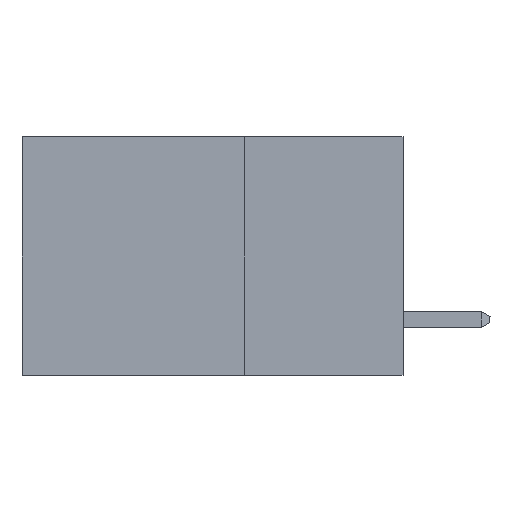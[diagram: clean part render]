
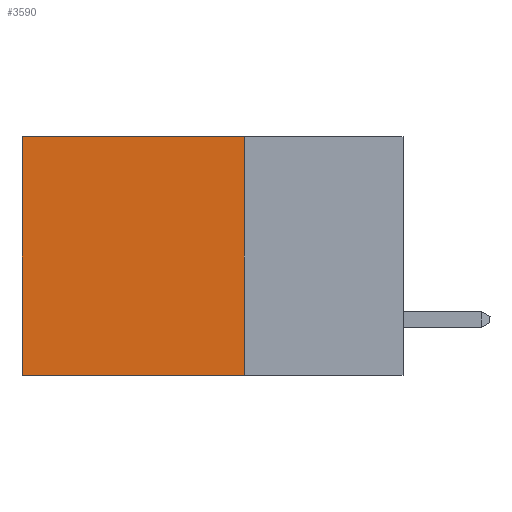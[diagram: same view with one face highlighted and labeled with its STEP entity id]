
A CAD part, left-side view. The second image highlights one B-rep face of the part: STEP entity #3590.
In plain terms, the highlighted planar face has unit normal (-1, 0, 0).
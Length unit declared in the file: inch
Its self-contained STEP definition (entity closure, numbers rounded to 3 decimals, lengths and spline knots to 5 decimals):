
#98 = VECTOR ( 'NONE', #6713, 39.37008 ) ;
#166 = VERTEX_POINT ( 'NONE', #9042 ) ;
#583 = LINE ( 'NONE', #1980, #8184 ) ;
#744 = VECTOR ( 'NONE', #755, 39.37008 ) ;
#755 = DIRECTION ( 'NONE',  ( 0., 0., -1. ) ) ;
#811 = EDGE_LOOP ( 'NONE', ( #7023, #7026, #1239, #4634 ) ) ;
#1239 = ORIENTED_EDGE ( 'NONE', *, *, #2025, .F. ) ;
#1556 = CARTESIAN_POINT ( 'NONE',  ( 0.2875, 0.25, -0.375 ) ) ;
#1712 = VERTEX_POINT ( 'NONE', #8568 ) ;
#1980 = CARTESIAN_POINT ( 'NONE',  ( 0.2875, 0.25, -0.375 ) ) ;
#2025 = EDGE_CURVE ( 'NONE', #3100, #166, #4269, .T. ) ;
#2081 = DIRECTION ( 'NONE',  ( 1., 0., 0. ) ) ;
#2112 = CARTESIAN_POINT ( 'NONE',  ( 0.2875, 0.6, -0.375 ) ) ;
#2979 = CARTESIAN_POINT ( 'NONE',  ( 0.2875, 0.25, 0. ) ) ;
#3008 = EDGE_CURVE ( 'NONE', #3100, #6334, #3666, .T. ) ;
#3100 = VERTEX_POINT ( 'NONE', #2979 ) ;
#3590 = ADVANCED_FACE ( 'NONE', ( #8355 ), #7936, .F. ) ;
#3645 = EDGE_CURVE ( 'NONE', #6334, #1712, #6968, .T. ) ;
#3666 = LINE ( 'NONE', #5583, #5613 ) ;
#4269 = LINE ( 'NONE', #1556, #98 ) ;
#4292 = CARTESIAN_POINT ( 'NONE',  ( 0.2875, 0.25, -0.375 ) ) ;
#4634 = ORIENTED_EDGE ( 'NONE', *, *, #3008, .T. ) ;
#5583 = CARTESIAN_POINT ( 'NONE',  ( 0.2875, 0.25, 0. ) ) ;
#5613 = VECTOR ( 'NONE', #7085, 39.37008 ) ;
#5998 = EDGE_CURVE ( 'NONE', #166, #1712, #583, .T. ) ;
#6334 = VERTEX_POINT ( 'NONE', #7626 ) ;
#6713 = DIRECTION ( 'NONE',  ( 0., 0., -1. ) ) ;
#6968 = LINE ( 'NONE', #2112, #744 ) ;
#7023 = ORIENTED_EDGE ( 'NONE', *, *, #3645, .T. ) ;
#7026 = ORIENTED_EDGE ( 'NONE', *, *, #5998, .F. ) ;
#7085 = DIRECTION ( 'NONE',  ( 0., 1., 0. ) ) ;
#7626 = CARTESIAN_POINT ( 'NONE',  ( 0.2875, 0.6, 0. ) ) ;
#7936 = PLANE ( 'NONE',  #8291 ) ;
#8184 = VECTOR ( 'NONE', #9463, 39.37008 ) ;
#8291 = AXIS2_PLACEMENT_3D ( 'NONE', #4292, #2081, #9435 ) ;
#8355 = FACE_OUTER_BOUND ( 'NONE', #811, .T. ) ;
#8568 = CARTESIAN_POINT ( 'NONE',  ( 0.2875, 0.6, -0.375 ) ) ;
#9042 = CARTESIAN_POINT ( 'NONE',  ( 0.2875, 0.25, -0.375 ) ) ;
#9435 = DIRECTION ( 'NONE',  ( 0., 0., -1. ) ) ;
#9463 = DIRECTION ( 'NONE',  ( 0., 1., 0. ) ) ;
